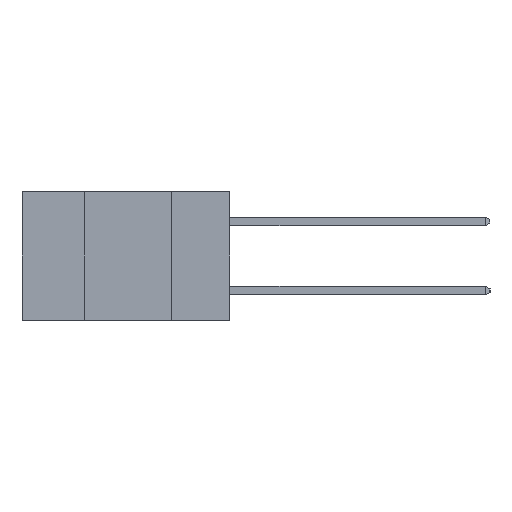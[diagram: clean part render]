
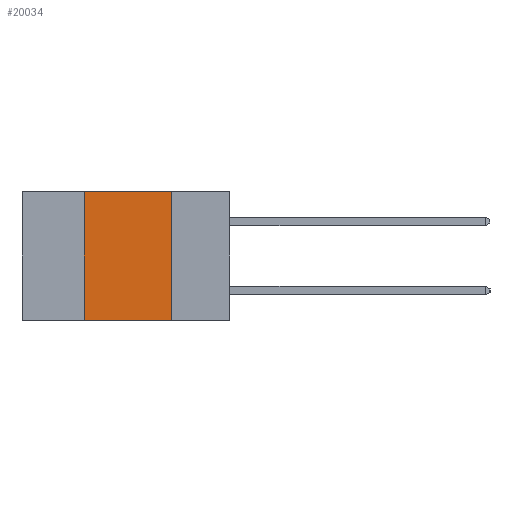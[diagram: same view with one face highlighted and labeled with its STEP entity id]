
A CAD part, left-side view. The second image highlights one B-rep face of the part: STEP entity #20034.
In plain terms, the highlighted planar face has unit normal (-1, 0, 0).
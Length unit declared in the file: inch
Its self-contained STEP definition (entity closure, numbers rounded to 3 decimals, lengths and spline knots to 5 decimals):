
#611 = LINE ( 'NONE', #23469, #21046 ) ;
#725 = CARTESIAN_POINT ( 'NONE',  ( 0., 0.42, -0.37 ) ) ;
#917 = EDGE_LOOP ( 'NONE', ( #10270, #19222, #10881, #9519 ) ) ;
#1936 = CARTESIAN_POINT ( 'NONE',  ( 0., 0.17, 0. ) ) ;
#2871 = DIRECTION ( 'NONE',  ( 0., 0., -1. ) ) ;
#3723 = DIRECTION ( 'NONE',  ( 0., -1., 0. ) ) ;
#4098 = EDGE_CURVE ( 'NONE', #17730, #17902, #14315, .T. ) ;
#4394 = VECTOR ( 'NONE', #10390, 39.37008 ) ;
#5670 = EDGE_CURVE ( 'NONE', #24992, #17730, #611, .T. ) ;
#7795 = FACE_OUTER_BOUND ( 'NONE', #917, .T. ) ;
#8216 = LINE ( 'NONE', #25308, #23388 ) ;
#8615 = EDGE_CURVE ( 'NONE', #15641, #17902, #8216, .T. ) ;
#9519 = ORIENTED_EDGE ( 'NONE', *, *, #8615, .T. ) ;
#9592 = CARTESIAN_POINT ( 'NONE',  ( 0., 0.42, -0.37 ) ) ;
#10270 = ORIENTED_EDGE ( 'NONE', *, *, #4098, .F. ) ;
#10390 = DIRECTION ( 'NONE',  ( 0., 0., -1. ) ) ;
#10421 = CARTESIAN_POINT ( 'NONE',  ( 0., 0.17, -0.37 ) ) ;
#10881 = ORIENTED_EDGE ( 'NONE', *, *, #13687, .F. ) ;
#12754 = PLANE ( 'NONE',  #12845 ) ;
#12845 = AXIS2_PLACEMENT_3D ( 'NONE', #24618, #14757, #2871 ) ;
#13464 = DIRECTION ( 'NONE',  ( 0., -1., 0. ) ) ;
#13687 = EDGE_CURVE ( 'NONE', #15641, #24992, #18073, .T. ) ;
#14315 = LINE ( 'NONE', #10421, #4394 ) ;
#14574 = DIRECTION ( 'NONE',  ( 0., 0., 1. ) ) ;
#14757 = DIRECTION ( 'NONE',  ( 1., 0., 0. ) ) ;
#15641 = VERTEX_POINT ( 'NONE', #9592 ) ;
#16268 = CARTESIAN_POINT ( 'NONE',  ( 0., 0.42, 0. ) ) ;
#17730 = VERTEX_POINT ( 'NONE', #1936 ) ;
#17902 = VERTEX_POINT ( 'NONE', #20301 ) ;
#18073 = LINE ( 'NONE', #725, #23317 ) ;
#19222 = ORIENTED_EDGE ( 'NONE', *, *, #5670, .F. ) ;
#20034 = ADVANCED_FACE ( 'NONE', ( #7795 ), #12754, .F. ) ;
#20301 = CARTESIAN_POINT ( 'NONE',  ( 0., 0.17, -0.37 ) ) ;
#21046 = VECTOR ( 'NONE', #3723, 39.37008 ) ;
#23317 = VECTOR ( 'NONE', #14574, 39.37008 ) ;
#23388 = VECTOR ( 'NONE', #13464, 39.37008 ) ;
#23469 = CARTESIAN_POINT ( 'NONE',  ( 0., 0.6, 0. ) ) ;
#24618 = CARTESIAN_POINT ( 'NONE',  ( 0., 0.6, 0. ) ) ;
#24992 = VERTEX_POINT ( 'NONE', #16268 ) ;
#25308 = CARTESIAN_POINT ( 'NONE',  ( 0., 0.6, -0.37 ) ) ;
